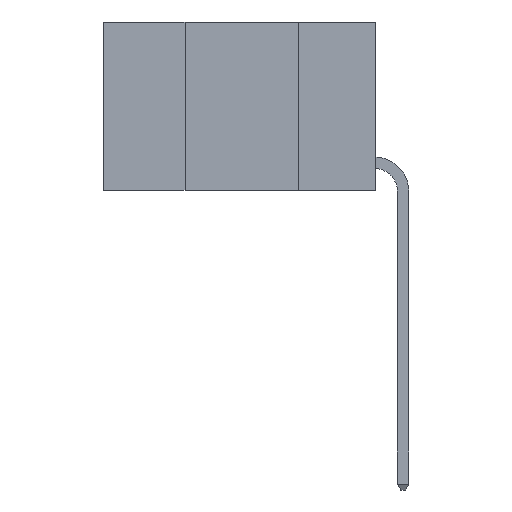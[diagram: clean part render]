
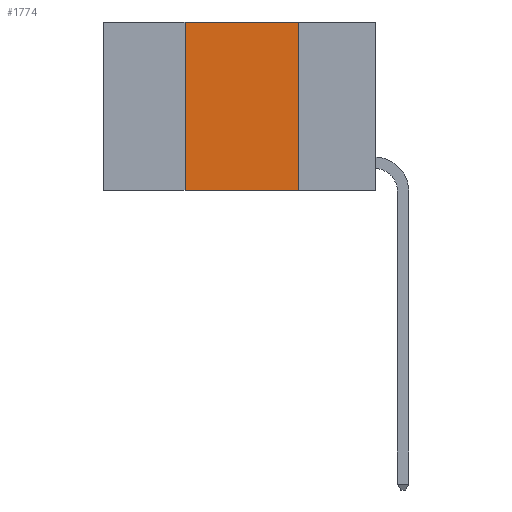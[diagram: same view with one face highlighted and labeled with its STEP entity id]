
A CAD part, left-side view. The second image highlights one B-rep face of the part: STEP entity #1774.
In plain terms, the highlighted planar face has unit normal (-1, 0, 0).
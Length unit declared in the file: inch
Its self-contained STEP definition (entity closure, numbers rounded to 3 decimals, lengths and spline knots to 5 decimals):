
#99 = ORIENTED_EDGE ( 'NONE', *, *, #758, .F. ) ;
#595 = VERTEX_POINT ( 'NONE', #1590 ) ;
#758 = EDGE_CURVE ( 'NONE', #3588, #8141, #2156, .T. ) ;
#1088 = CARTESIAN_POINT ( 'NONE',  ( 0., 0.42, 0. ) ) ;
#1412 = EDGE_CURVE ( 'NONE', #2742, #595, #5388, .T. ) ;
#1452 = EDGE_LOOP ( 'NONE', ( #9273, #99, #2376, #3058 ) ) ;
#1496 = LINE ( 'NONE', #6730, #3256 ) ;
#1590 = CARTESIAN_POINT ( 'NONE',  ( 0., 0.17, -0.37 ) ) ;
#1774 = ADVANCED_FACE ( 'NONE', ( #2587 ), #7180, .F. ) ;
#2156 = LINE ( 'NONE', #8861, #7542 ) ;
#2264 = CARTESIAN_POINT ( 'NONE',  ( 0., 0.6, 0. ) ) ;
#2376 = ORIENTED_EDGE ( 'NONE', *, *, #7169, .F. ) ;
#2587 = FACE_OUTER_BOUND ( 'NONE', #1452, .T. ) ;
#2604 = EDGE_CURVE ( 'NONE', #8141, #595, #3556, .T. ) ;
#2742 = VERTEX_POINT ( 'NONE', #3369 ) ;
#3058 = ORIENTED_EDGE ( 'NONE', *, *, #1412, .T. ) ;
#3254 = DIRECTION ( 'NONE',  ( 0., 0., 1. ) ) ;
#3256 = VECTOR ( 'NONE', #3254, 39.37008 ) ;
#3369 = CARTESIAN_POINT ( 'NONE',  ( 0., 0.42, -0.37 ) ) ;
#3556 = LINE ( 'NONE', #8800, #7056 ) ;
#3588 = VERTEX_POINT ( 'NONE', #1088 ) ;
#3693 = DIRECTION ( 'NONE',  ( 0., 0., -1. ) ) ;
#4030 = DIRECTION ( 'NONE',  ( 0., -1., 0. ) ) ;
#4933 = CARTESIAN_POINT ( 'NONE',  ( 0., 0.17, 0. ) ) ;
#5388 = LINE ( 'NONE', #7522, #8752 ) ;
#5975 = DIRECTION ( 'NONE',  ( 0., -1., 0. ) ) ;
#6581 = AXIS2_PLACEMENT_3D ( 'NONE', #2264, #7895, #3693 ) ;
#6730 = CARTESIAN_POINT ( 'NONE',  ( 0., 0.42, 0. ) ) ;
#7056 = VECTOR ( 'NONE', #8103, 39.37008 ) ;
#7169 = EDGE_CURVE ( 'NONE', #2742, #3588, #1496, .T. ) ;
#7180 = PLANE ( 'NONE',  #6581 ) ;
#7522 = CARTESIAN_POINT ( 'NONE',  ( 0., 0.6, -0.37 ) ) ;
#7542 = VECTOR ( 'NONE', #5975, 39.37008 ) ;
#7895 = DIRECTION ( 'NONE',  ( 1., 0., 0. ) ) ;
#8103 = DIRECTION ( 'NONE',  ( 0., 0., -1. ) ) ;
#8141 = VERTEX_POINT ( 'NONE', #4933 ) ;
#8752 = VECTOR ( 'NONE', #4030, 39.37008 ) ;
#8800 = CARTESIAN_POINT ( 'NONE',  ( 0., 0.17, 0. ) ) ;
#8861 = CARTESIAN_POINT ( 'NONE',  ( 0., 0.6, 0. ) ) ;
#9273 = ORIENTED_EDGE ( 'NONE', *, *, #2604, .F. ) ;
